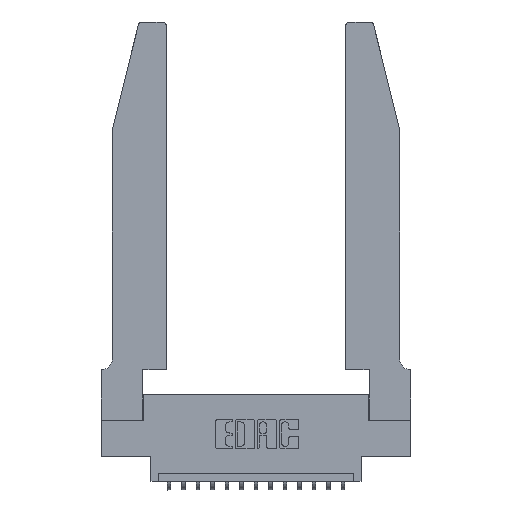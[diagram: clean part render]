
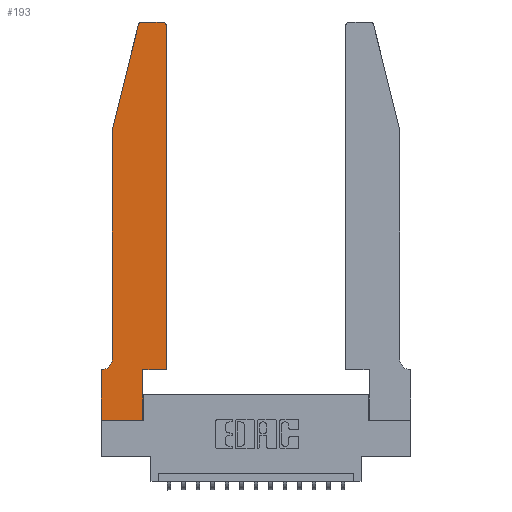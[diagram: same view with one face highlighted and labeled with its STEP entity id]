
A CAD part, top view. The second image highlights one B-rep face of the part: STEP entity #193.
In plain terms, the highlighted planar face has unit normal (0, 0, 1).
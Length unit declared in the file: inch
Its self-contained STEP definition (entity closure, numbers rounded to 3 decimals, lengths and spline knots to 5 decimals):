
#10 = VERTEX_POINT ( 'NONE', #12402 ) ;
#193 = ADVANCED_FACE ( 'NONE', ( #4802 ), #16158, .T. ) ;
#267 = VECTOR ( 'NONE', #13756, 39.37008 ) ;
#322 = CIRCLE ( 'NONE', #14856, 0.03 ) ;
#449 = EDGE_CURVE ( 'NONE', #2703, #18146, #16963, .T. ) ;
#764 = ORIENTED_EDGE ( 'NONE', *, *, #5878, .T. ) ;
#1462 = ORIENTED_EDGE ( 'NONE', *, *, #5268, .T. ) ;
#1479 = CARTESIAN_POINT ( 'NONE',  ( 0.4505, 0.35, 0.37 ) ) ;
#1528 = DIRECTION ( 'NONE',  ( 0., 0., -1. ) ) ;
#2000 = ORIENTED_EDGE ( 'NONE', *, *, #10945, .T. ) ;
#2110 = DIRECTION ( 'NONE',  ( -0.239, -0.971, 0. ) ) ;
#2195 = AXIS2_PLACEMENT_3D ( 'NONE', #14514, #17324, #8841 ) ;
#2220 = ORIENTED_EDGE ( 'NONE', *, *, #4905, .T. ) ;
#2512 = VECTOR ( 'NONE', #17678, 39.37008 ) ;
#2643 = EDGE_CURVE ( 'NONE', #5454, #18249, #6318, .T. ) ;
#2703 = VERTEX_POINT ( 'NONE', #7739 ) ;
#2739 = EDGE_CURVE ( 'NONE', #8084, #5454, #2935, .T. ) ;
#2928 = DIRECTION ( 'NONE',  ( 1., 0., 0. ) ) ;
#2935 = LINE ( 'NONE', #16375, #8356 ) ;
#3435 = VERTEX_POINT ( 'NONE', #11006 ) ;
#3599 = CARTESIAN_POINT ( 'NONE',  ( 0., 0., 0.37 ) ) ;
#3667 = CARTESIAN_POINT ( 'NONE',  ( 0.4505, 0.35, 0.37 ) ) ;
#3694 = VECTOR ( 'NONE', #11044, 39.37008 ) ;
#4087 = LINE ( 'NONE', #13080, #17820 ) ;
#4293 = CARTESIAN_POINT ( 'NONE',  ( 0., 0.35, 0.37 ) ) ;
#4484 = DIRECTION ( 'NONE',  ( -1., 0., 0. ) ) ;
#4636 = EDGE_LOOP ( 'NONE', ( #764, #2000, #5440, #1462, #8275, #16440, #9959, #17354, #18096, #2220, #4684, #17898 ) ) ;
#4684 = ORIENTED_EDGE ( 'NONE', *, *, #15532, .T. ) ;
#4802 = FACE_OUTER_BOUND ( 'NONE', #4636, .T. ) ;
#4905 = EDGE_CURVE ( 'NONE', #16129, #13709, #7955, .T. ) ;
#4933 = DIRECTION ( 'NONE',  ( 0., -1., 0. ) ) ;
#5213 = DIRECTION ( 'NONE',  ( 0., 0., 1. ) ) ;
#5268 = EDGE_CURVE ( 'NONE', #3435, #10, #7260, .T. ) ;
#5274 = DIRECTION ( 'NONE',  ( 1., 0., 0. ) ) ;
#5440 = ORIENTED_EDGE ( 'NONE', *, *, #8832, .T. ) ;
#5454 = VERTEX_POINT ( 'NONE', #16698 ) ;
#5494 = AXIS2_PLACEMENT_3D ( 'NONE', #10875, #5213, #5274 ) ;
#5865 = VECTOR ( 'NONE', #9234, 39.37008 ) ;
#5878 = EDGE_CURVE ( 'NONE', #18146, #8343, #8131, .T. ) ;
#6137 = VECTOR ( 'NONE', #2928, 39.37008 ) ;
#6315 = CARTESIAN_POINT ( 'NONE',  ( 0.0755, 0.35, 0.37 ) ) ;
#6318 = LINE ( 'NONE', #3599, #5865 ) ;
#6931 = LINE ( 'NONE', #12232, #12993 ) ;
#7033 = CARTESIAN_POINT ( 'NONE',  ( 0.284, 2.72, 0.37 ) ) ;
#7260 = LINE ( 'NONE', #7618, #2512 ) ;
#7618 = CARTESIAN_POINT ( 'NONE',  ( 0.0755, 2., 0.37 ) ) ;
#7739 = CARTESIAN_POINT ( 'NONE',  ( 0.4505, 2.72, 0.37 ) ) ;
#7955 = LINE ( 'NONE', #1479, #6137 ) ;
#8084 = VERTEX_POINT ( 'NONE', #4293 ) ;
#8131 = LINE ( 'NONE', #18018, #15751 ) ;
#8275 = ORIENTED_EDGE ( 'NONE', *, *, #13718, .T. ) ;
#8343 = VERTEX_POINT ( 'NONE', #11738 ) ;
#8356 = VECTOR ( 'NONE', #4933, 39.37008 ) ;
#8470 = DIRECTION ( 'NONE',  ( 1., 0., 0. ) ) ;
#8832 = EDGE_CURVE ( 'NONE', #10459, #3435, #6931, .T. ) ;
#8841 = DIRECTION ( 'NONE',  ( 1., 0., 0. ) ) ;
#9234 = DIRECTION ( 'NONE',  ( 1., 0., 0. ) ) ;
#9304 = DIRECTION ( 'NONE',  ( 0., 1., 0. ) ) ;
#9361 = LINE ( 'NONE', #3667, #3694 ) ;
#9959 = ORIENTED_EDGE ( 'NONE', *, *, #2739, .T. ) ;
#10459 = VERTEX_POINT ( 'NONE', #15753 ) ;
#10875 = CARTESIAN_POINT ( 'NONE',  ( 0.4205, 2.72, 0.37 ) ) ;
#10930 = AXIS2_PLACEMENT_3D ( 'NONE', #14226, #1528, #4484 ) ;
#10945 = EDGE_CURVE ( 'NONE', #8343, #10459, #322, .T. ) ;
#11006 = CARTESIAN_POINT ( 'NONE',  ( 0.0755, 2., 0.37 ) ) ;
#11044 = DIRECTION ( 'NONE',  ( 0., 1., 0. ) ) ;
#11525 = VERTEX_POINT ( 'NONE', #17889 ) ;
#11726 = LINE ( 'NONE', #6315, #267 ) ;
#11738 = CARTESIAN_POINT ( 'NONE',  ( 0.284, 2.75, 0.37 ) ) ;
#12232 = CARTESIAN_POINT ( 'NONE',  ( 0.0755, 2., 0.37 ) ) ;
#12402 = CARTESIAN_POINT ( 'NONE',  ( 0.0755, 0.42, 0.37 ) ) ;
#12806 = CARTESIAN_POINT ( 'NONE',  ( 0.4505, 0.35, 0.37 ) ) ;
#12993 = VECTOR ( 'NONE', #2110, 39.37008 ) ;
#13080 = CARTESIAN_POINT ( 'NONE',  ( 0.2865, 0.35, 0.37 ) ) ;
#13709 = VERTEX_POINT ( 'NONE', #12806 ) ;
#13718 = EDGE_CURVE ( 'NONE', #10, #11525, #13880, .T. ) ;
#13756 = DIRECTION ( 'NONE',  ( -1., 0., 0. ) ) ;
#13880 = CIRCLE ( 'NONE', #10930, 0.07 ) ;
#14226 = CARTESIAN_POINT ( 'NONE',  ( 0.0055, 0.42, 0.37 ) ) ;
#14440 = DIRECTION ( 'NONE',  ( -1., 0., 0. ) ) ;
#14514 = CARTESIAN_POINT ( 'NONE',  ( 0., 0.35, 0.37 ) ) ;
#14531 = CARTESIAN_POINT ( 'NONE',  ( 0.2865, 0., 0.37 ) ) ;
#14586 = CARTESIAN_POINT ( 'NONE',  ( 0.2865, 0.35, 0.37 ) ) ;
#14856 = AXIS2_PLACEMENT_3D ( 'NONE', #7033, #17088, #8470 ) ;
#15532 = EDGE_CURVE ( 'NONE', #13709, #2703, #9361, .T. ) ;
#15751 = VECTOR ( 'NONE', #14440, 39.37008 ) ;
#15753 = CARTESIAN_POINT ( 'NONE',  ( 0.25487, 2.72718, 0.37 ) ) ;
#16129 = VERTEX_POINT ( 'NONE', #14586 ) ;
#16158 = PLANE ( 'NONE',  #2195 ) ;
#16375 = CARTESIAN_POINT ( 'NONE',  ( 0., 0., 0.37 ) ) ;
#16440 = ORIENTED_EDGE ( 'NONE', *, *, #18540, .T. ) ;
#16698 = CARTESIAN_POINT ( 'NONE',  ( 0., 0., 0.37 ) ) ;
#16963 = CIRCLE ( 'NONE', #5494, 0.03 ) ;
#17088 = DIRECTION ( 'NONE',  ( 0., 0., 1. ) ) ;
#17324 = DIRECTION ( 'NONE',  ( 0., 0., 1. ) ) ;
#17354 = ORIENTED_EDGE ( 'NONE', *, *, #2643, .T. ) ;
#17678 = DIRECTION ( 'NONE',  ( 0., -1., 0. ) ) ;
#17820 = VECTOR ( 'NONE', #9304, 39.37008 ) ;
#17889 = CARTESIAN_POINT ( 'NONE',  ( 0.0055, 0.35, 0.37 ) ) ;
#17898 = ORIENTED_EDGE ( 'NONE', *, *, #449, .T. ) ;
#17917 = EDGE_CURVE ( 'NONE', #18249, #16129, #4087, .T. ) ;
#18018 = CARTESIAN_POINT ( 'NONE',  ( 0.2605, 2.75, 0.37 ) ) ;
#18096 = ORIENTED_EDGE ( 'NONE', *, *, #17917, .T. ) ;
#18146 = VERTEX_POINT ( 'NONE', #18378 ) ;
#18249 = VERTEX_POINT ( 'NONE', #14531 ) ;
#18378 = CARTESIAN_POINT ( 'NONE',  ( 0.4205, 2.75, 0.37 ) ) ;
#18540 = EDGE_CURVE ( 'NONE', #11525, #8084, #11726, .T. ) ;
